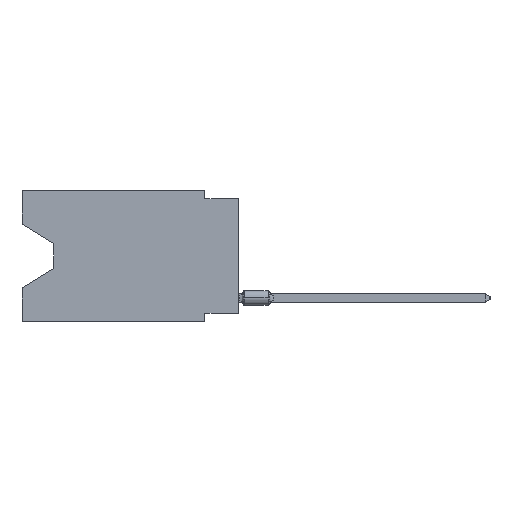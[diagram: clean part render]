
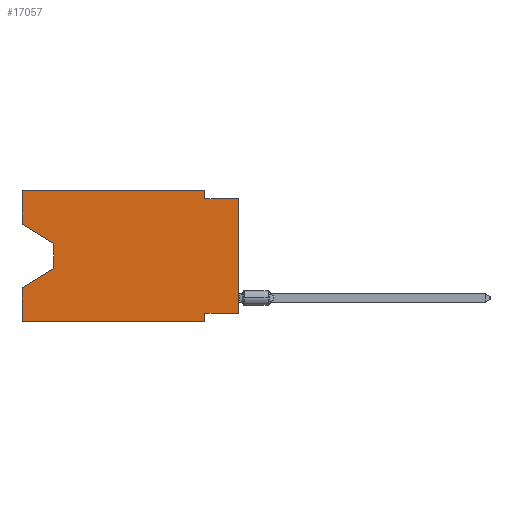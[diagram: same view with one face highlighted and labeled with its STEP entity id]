
A CAD part, left-side view. The second image highlights one B-rep face of the part: STEP entity #17057.
In plain terms, the highlighted planar face has unit normal (-1, 0, 0).
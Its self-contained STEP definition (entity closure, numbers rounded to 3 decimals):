
#437 = ORIENTED_EDGE ( 'NONE', *, *, #86881, .F. ) ;
#559 = LINE ( 'NONE', #15705, #46536 ) ;
#2355 = LINE ( 'NONE', #23296, #33705 ) ;
#4134 = EDGE_CURVE ( 'NONE', #13856, #78671, #60587, .T. ) ;
#6723 = CARTESIAN_POINT ( 'NONE',  ( 0., 16.383, 0. ) ) ;
#7317 = VERTEX_POINT ( 'NONE', #85496 ) ;
#8451 = ORIENTED_EDGE ( 'NONE', *, *, #87813, .F. ) ;
#9433 = ORIENTED_EDGE ( 'NONE', *, *, #67821, .F. ) ;
#10677 = LINE ( 'NONE', #84664, #61970 ) ;
#11165 = DIRECTION ( 'NONE',  ( 0., -1., 0. ) ) ;
#12366 = ORIENTED_EDGE ( 'NONE', *, *, #53076, .T. ) ;
#13148 = VECTOR ( 'NONE', #14752, 1000. ) ;
#13856 = VERTEX_POINT ( 'NONE', #86522 ) ;
#14091 = LINE ( 'NONE', #76046, #21328 ) ;
#14661 = DIRECTION ( 'NONE',  ( 0., 0., -1. ) ) ;
#14752 = DIRECTION ( 'NONE',  ( 0., 0., -1. ) ) ;
#15163 = VERTEX_POINT ( 'NONE', #51396 ) ;
#15548 = VECTOR ( 'NONE', #74918, 1000. ) ;
#15705 = CARTESIAN_POINT ( 'NONE',  ( 0., 0., 0. ) ) ;
#17057 = ADVANCED_FACE ( 'NONE', ( #76622 ), #60288, .F. ) ;
#17605 = VERTEX_POINT ( 'NONE', #78281 ) ;
#17667 = ORIENTED_EDGE ( 'NONE', *, *, #32467, .F. ) ;
#19196 = VERTEX_POINT ( 'NONE', #46890 ) ;
#19417 = DIRECTION ( 'NONE',  ( 0., -1., 0. ) ) ;
#19846 = VERTEX_POINT ( 'NONE', #50173 ) ;
#21328 = VECTOR ( 'NONE', #76923, 1000. ) ;
#21826 = VECTOR ( 'NONE', #19417, 1000. ) ;
#23296 = CARTESIAN_POINT ( 'NONE',  ( 0., 13.97, -4.013 ) ) ;
#26480 = CARTESIAN_POINT ( 'NONE',  ( 0., 0., -9.271 ) ) ;
#27334 = DIRECTION ( 'NONE',  ( 0., 0., -1. ) ) ;
#27530 = AXIS2_PLACEMENT_3D ( 'NONE', #46502, #83299, #14661 ) ;
#28194 = LINE ( 'NONE', #70068, #70878 ) ;
#30875 = VECTOR ( 'NONE', #45022, 1000. ) ;
#30991 = ORIENTED_EDGE ( 'NONE', *, *, #4134, .T. ) ;
#31948 = ORIENTED_EDGE ( 'NONE', *, *, #60120, .F. ) ;
#32467 = EDGE_CURVE ( 'NONE', #15163, #17605, #67041, .T. ) ;
#33705 = VECTOR ( 'NONE', #56710, 1000. ) ;
#33823 = EDGE_CURVE ( 'NONE', #7317, #19196, #14091, .T. ) ;
#35326 = VECTOR ( 'NONE', #51808, 1000. ) ;
#37005 = DIRECTION ( 'NONE',  ( 0., -0.855, -0.519 ) ) ;
#37533 = DIRECTION ( 'NONE',  ( 0., 0., 1. ) ) ;
#39169 = VERTEX_POINT ( 'NONE', #60097 ) ;
#39976 = CARTESIAN_POINT ( 'NONE',  ( 0., 2.54, -9.271 ) ) ;
#40474 = ORIENTED_EDGE ( 'NONE', *, *, #33823, .T. ) ;
#45022 = DIRECTION ( 'NONE',  ( 0., 0., 1. ) ) ;
#45047 = CARTESIAN_POINT ( 'NONE',  ( 0., 16.383, -9.906 ) ) ;
#45473 = CARTESIAN_POINT ( 'NONE',  ( 0., 16.383, 0. ) ) ;
#46502 = CARTESIAN_POINT ( 'NONE',  ( 0., 16.383, 0. ) ) ;
#46536 = VECTOR ( 'NONE', #37533, 1000. ) ;
#46557 = CARTESIAN_POINT ( 'NONE',  ( 0., 2.54, 0. ) ) ;
#46890 = CARTESIAN_POINT ( 'NONE',  ( 0., 16.383, -7.36 ) ) ;
#50173 = CARTESIAN_POINT ( 'NONE',  ( 0., 0., -0.635 ) ) ;
#51396 = CARTESIAN_POINT ( 'NONE',  ( 0., 2.54, 0. ) ) ;
#51808 = DIRECTION ( 'NONE',  ( 0., 1., 0. ) ) ;
#52171 = EDGE_LOOP ( 'NONE', ( #78022, #12366, #40474, #437, #30991, #31948, #82421, #81963, #64571, #17667, #9433, #8451 ) ) ;
#53076 = EDGE_CURVE ( 'NONE', #81848, #7317, #2355, .T. ) ;
#55436 = LINE ( 'NONE', #60834, #21826 ) ;
#55760 = CARTESIAN_POINT ( 'NONE',  ( 0., 2.54, -9.906 ) ) ;
#56164 = VERTEX_POINT ( 'NONE', #26480 ) ;
#56199 = LINE ( 'NONE', #55760, #13148 ) ;
#56710 = DIRECTION ( 'NONE',  ( 0., 0., -1. ) ) ;
#57045 = LINE ( 'NONE', #58367, #30875 ) ;
#58057 = CARTESIAN_POINT ( 'NONE',  ( 0., 0., -9.271 ) ) ;
#58367 = CARTESIAN_POINT ( 'NONE',  ( 0., 16.383, 0. ) ) ;
#60097 = CARTESIAN_POINT ( 'NONE',  ( 0., 16.383, -2.546 ) ) ;
#60120 = EDGE_CURVE ( 'NONE', #83766, #78671, #56199, .T. ) ;
#60288 = PLANE ( 'NONE',  #27530 ) ;
#60587 = LINE ( 'NONE', #45047, #81557 ) ;
#60834 = CARTESIAN_POINT ( 'NONE',  ( 0., 0., -0.635 ) ) ;
#61617 = DIRECTION ( 'NONE',  ( 0., 0., 1. ) ) ;
#61970 = VECTOR ( 'NONE', #37005, 1000. ) ;
#64571 = ORIENTED_EDGE ( 'NONE', *, *, #73734, .F. ) ;
#66068 = LINE ( 'NONE', #58057, #35326 ) ;
#66073 = CARTESIAN_POINT ( 'NONE',  ( 0., 13.97, -4.013 ) ) ;
#66261 = EDGE_CURVE ( 'NONE', #56164, #19846, #559, .T. ) ;
#67041 = LINE ( 'NONE', #46557, #86555 ) ;
#67821 = EDGE_CURVE ( 'NONE', #82311, #15163, #69090, .T. ) ;
#69090 = LINE ( 'NONE', #6723, #15548 ) ;
#70068 = CARTESIAN_POINT ( 'NONE',  ( 0., 16.383, 0. ) ) ;
#70878 = VECTOR ( 'NONE', #61617, 1000. ) ;
#73734 = EDGE_CURVE ( 'NONE', #17605, #19846, #55436, .T. ) ;
#73859 = CARTESIAN_POINT ( 'NONE',  ( 0., 2.54, -9.906 ) ) ;
#74918 = DIRECTION ( 'NONE',  ( 0., -1., 0. ) ) ;
#76046 = CARTESIAN_POINT ( 'NONE',  ( 0., 13.97, -5.893 ) ) ;
#76622 = FACE_OUTER_BOUND ( 'NONE', #52171, .T. ) ;
#76923 = DIRECTION ( 'NONE',  ( 0., 0.855, -0.519 ) ) ;
#78022 = ORIENTED_EDGE ( 'NONE', *, *, #85734, .T. ) ;
#78238 = EDGE_CURVE ( 'NONE', #56164, #83766, #66068, .T. ) ;
#78281 = CARTESIAN_POINT ( 'NONE',  ( 0., 2.54, -0.635 ) ) ;
#78671 = VERTEX_POINT ( 'NONE', #73859 ) ;
#81557 = VECTOR ( 'NONE', #11165, 1000. ) ;
#81848 = VERTEX_POINT ( 'NONE', #66073 ) ;
#81963 = ORIENTED_EDGE ( 'NONE', *, *, #66261, .T. ) ;
#82311 = VERTEX_POINT ( 'NONE', #45473 ) ;
#82421 = ORIENTED_EDGE ( 'NONE', *, *, #78238, .F. ) ;
#83299 = DIRECTION ( 'NONE',  ( 1., 0., 0. ) ) ;
#83766 = VERTEX_POINT ( 'NONE', #39976 ) ;
#84664 = CARTESIAN_POINT ( 'NONE',  ( 0., 16.383, -2.546 ) ) ;
#85496 = CARTESIAN_POINT ( 'NONE',  ( 0., 13.97, -5.893 ) ) ;
#85734 = EDGE_CURVE ( 'NONE', #39169, #81848, #10677, .T. ) ;
#86522 = CARTESIAN_POINT ( 'NONE',  ( 0., 16.383, -9.906 ) ) ;
#86555 = VECTOR ( 'NONE', #27334, 1000. ) ;
#86881 = EDGE_CURVE ( 'NONE', #13856, #19196, #57045, .T. ) ;
#87813 = EDGE_CURVE ( 'NONE', #39169, #82311, #28194, .T. ) ;
